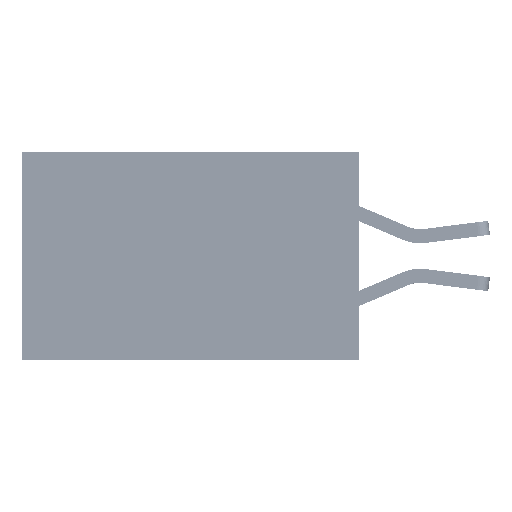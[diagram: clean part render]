
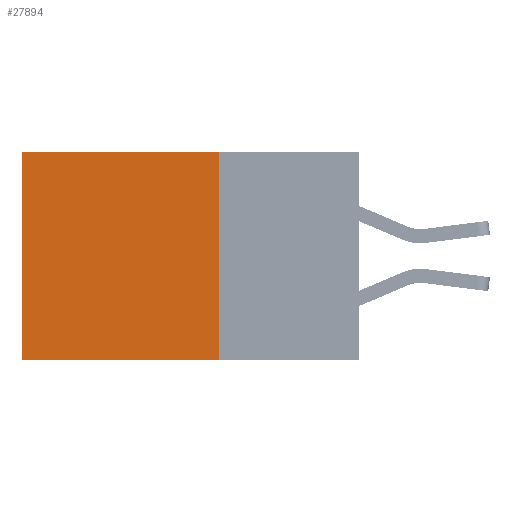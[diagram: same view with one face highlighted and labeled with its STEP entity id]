
A CAD part, left-side view. The second image highlights one B-rep face of the part: STEP entity #27894.
In plain terms, the highlighted planar face has unit normal (-1, 0, 0).
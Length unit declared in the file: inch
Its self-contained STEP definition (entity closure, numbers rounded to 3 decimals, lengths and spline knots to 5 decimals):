
#811 = CARTESIAN_POINT ( 'NONE',  ( 0.2875, 0.6, -0.37 ) ) ;
#6291 = LINE ( 'NONE', #28393, #25686 ) ;
#7582 = EDGE_CURVE ( 'NONE', #13507, #33683, #27654, .T. ) ;
#8887 = CARTESIAN_POINT ( 'NONE',  ( 0.2875, 0.6, 0. ) ) ;
#11397 = CARTESIAN_POINT ( 'NONE',  ( 0.2875, 0.25, 0. ) ) ;
#12010 = VECTOR ( 'NONE', #21927, 39.37008 ) ;
#13507 = VERTEX_POINT ( 'NONE', #11397 ) ;
#14024 = ORIENTED_EDGE ( 'NONE', *, *, #7582, .T. ) ;
#18290 = VECTOR ( 'NONE', #40201, 39.37008 ) ;
#21927 = DIRECTION ( 'NONE',  ( 0., 1., 0. ) ) ;
#22629 = VERTEX_POINT ( 'NONE', #40874 ) ;
#23355 = DIRECTION ( 'NONE',  ( 0., 1., 0. ) ) ;
#23700 = DIRECTION ( 'NONE',  ( 0., 0., -1. ) ) ;
#24740 = CARTESIAN_POINT ( 'NONE',  ( 0.2875, 0.25, 0. ) ) ;
#25686 = VECTOR ( 'NONE', #23355, 39.37008 ) ;
#25739 = DIRECTION ( 'NONE',  ( 0., 0., -1. ) ) ;
#27188 = ORIENTED_EDGE ( 'NONE', *, *, #32167, .F. ) ;
#27654 = LINE ( 'NONE', #24740, #12010 ) ;
#27721 = VERTEX_POINT ( 'NONE', #811 ) ;
#27894 = ADVANCED_FACE ( 'NONE', ( #44806 ), #37206, .F. ) ;
#28273 = VECTOR ( 'NONE', #23700, 39.37008 ) ;
#28393 = CARTESIAN_POINT ( 'NONE',  ( 0.2875, 0.25, -0.37 ) ) ;
#32167 = EDGE_CURVE ( 'NONE', #22629, #27721, #6291, .T. ) ;
#33382 = CARTESIAN_POINT ( 'NONE',  ( 0.2875, 0.25, 0. ) ) ;
#33683 = VERTEX_POINT ( 'NONE', #8887 ) ;
#34080 = EDGE_CURVE ( 'NONE', #13507, #22629, #38846, .T. ) ;
#34188 = EDGE_CURVE ( 'NONE', #33683, #27721, #41926, .T. ) ;
#37206 = PLANE ( 'NONE',  #45858 ) ;
#38846 = LINE ( 'NONE', #50980, #28273 ) ;
#39243 = ORIENTED_EDGE ( 'NONE', *, *, #34188, .T. ) ;
#40201 = DIRECTION ( 'NONE',  ( 0., 0., -1. ) ) ;
#40874 = CARTESIAN_POINT ( 'NONE',  ( 0.2875, 0.25, -0.37 ) ) ;
#41377 = DIRECTION ( 'NONE',  ( 1., 0., 0. ) ) ;
#41446 = ORIENTED_EDGE ( 'NONE', *, *, #34080, .F. ) ;
#41926 = LINE ( 'NONE', #48346, #18290 ) ;
#44806 = FACE_OUTER_BOUND ( 'NONE', #47449, .T. ) ;
#45858 = AXIS2_PLACEMENT_3D ( 'NONE', #33382, #41377, #25739 ) ;
#47449 = EDGE_LOOP ( 'NONE', ( #39243, #27188, #41446, #14024 ) ) ;
#48346 = CARTESIAN_POINT ( 'NONE',  ( 0.2875, 0.6, 0. ) ) ;
#50980 = CARTESIAN_POINT ( 'NONE',  ( 0.2875, 0.25, 0. ) ) ;
